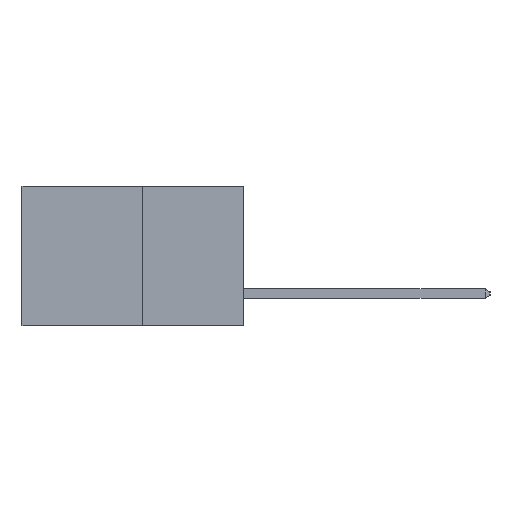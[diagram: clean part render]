
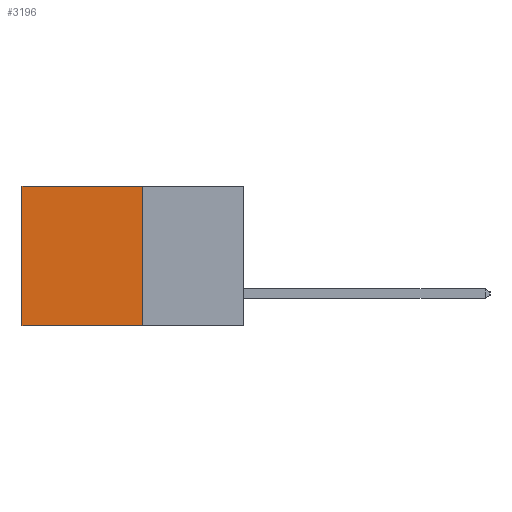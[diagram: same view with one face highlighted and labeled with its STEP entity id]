
A CAD part, left-side view. The second image highlights one B-rep face of the part: STEP entity #3196.
In plain terms, the highlighted planar face has unit normal (-1, 0, 0).
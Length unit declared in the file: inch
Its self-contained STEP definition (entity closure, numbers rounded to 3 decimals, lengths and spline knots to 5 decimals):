
#233 = CARTESIAN_POINT ( 'NONE',  ( 0.277, 0.27, -0.37 ) ) ;
#819 = EDGE_LOOP ( 'NONE', ( #5893, #14818, #8666, #2243 ) ) ;
#1605 = EDGE_CURVE ( 'NONE', #12141, #9554, #8541, .T. ) ;
#1995 = DIRECTION ( 'NONE',  ( 0., 0., -1. ) ) ;
#2243 = ORIENTED_EDGE ( 'NONE', *, *, #4330, .T. ) ;
#3196 = ADVANCED_FACE ( 'NONE', ( #4479 ), #13504, .F. ) ;
#3480 = VECTOR ( 'NONE', #8907, 39.37008 ) ;
#4330 = EDGE_CURVE ( 'NONE', #6852, #12141, #7840, .T. ) ;
#4374 = CARTESIAN_POINT ( 'NONE',  ( 0.277, 0.59, 0. ) ) ;
#4479 = FACE_OUTER_BOUND ( 'NONE', #819, .T. ) ;
#4574 = EDGE_CURVE ( 'NONE', #6852, #10259, #6901, .T. ) ;
#5362 = VECTOR ( 'NONE', #11385, 39.37008 ) ;
#5893 = ORIENTED_EDGE ( 'NONE', *, *, #1605, .T. ) ;
#6852 = VERTEX_POINT ( 'NONE', #8778 ) ;
#6901 = LINE ( 'NONE', #233, #9641 ) ;
#6941 = CARTESIAN_POINT ( 'NONE',  ( 0.277, 0.59, -0.37 ) ) ;
#7380 = AXIS2_PLACEMENT_3D ( 'NONE', #14188, #14086, #11258 ) ;
#7840 = LINE ( 'NONE', #9010, #3480 ) ;
#8541 = LINE ( 'NONE', #6941, #5362 ) ;
#8663 = LINE ( 'NONE', #10583, #14434 ) ;
#8666 = ORIENTED_EDGE ( 'NONE', *, *, #4574, .F. ) ;
#8778 = CARTESIAN_POINT ( 'NONE',  ( 0.277, 0.27, 0. ) ) ;
#8907 = DIRECTION ( 'NONE',  ( 0., 1., 0. ) ) ;
#9010 = CARTESIAN_POINT ( 'NONE',  ( 0.277, 0.27, 0. ) ) ;
#9383 = DIRECTION ( 'NONE',  ( 0., 1., 0. ) ) ;
#9554 = VERTEX_POINT ( 'NONE', #11108 ) ;
#9641 = VECTOR ( 'NONE', #1995, 39.37008 ) ;
#10259 = VERTEX_POINT ( 'NONE', #12299 ) ;
#10583 = CARTESIAN_POINT ( 'NONE',  ( 0.277, 0.27, -0.37 ) ) ;
#11108 = CARTESIAN_POINT ( 'NONE',  ( 0.277, 0.59, -0.37 ) ) ;
#11258 = DIRECTION ( 'NONE',  ( 0., 0., -1. ) ) ;
#11385 = DIRECTION ( 'NONE',  ( 0., 0., -1. ) ) ;
#11795 = EDGE_CURVE ( 'NONE', #10259, #9554, #8663, .T. ) ;
#12141 = VERTEX_POINT ( 'NONE', #4374 ) ;
#12299 = CARTESIAN_POINT ( 'NONE',  ( 0.277, 0.27, -0.37 ) ) ;
#13504 = PLANE ( 'NONE',  #7380 ) ;
#14086 = DIRECTION ( 'NONE',  ( 1., 0., 0. ) ) ;
#14188 = CARTESIAN_POINT ( 'NONE',  ( 0.277, 0.27, -0.37 ) ) ;
#14434 = VECTOR ( 'NONE', #9383, 39.37008 ) ;
#14818 = ORIENTED_EDGE ( 'NONE', *, *, #11795, .F. ) ;
